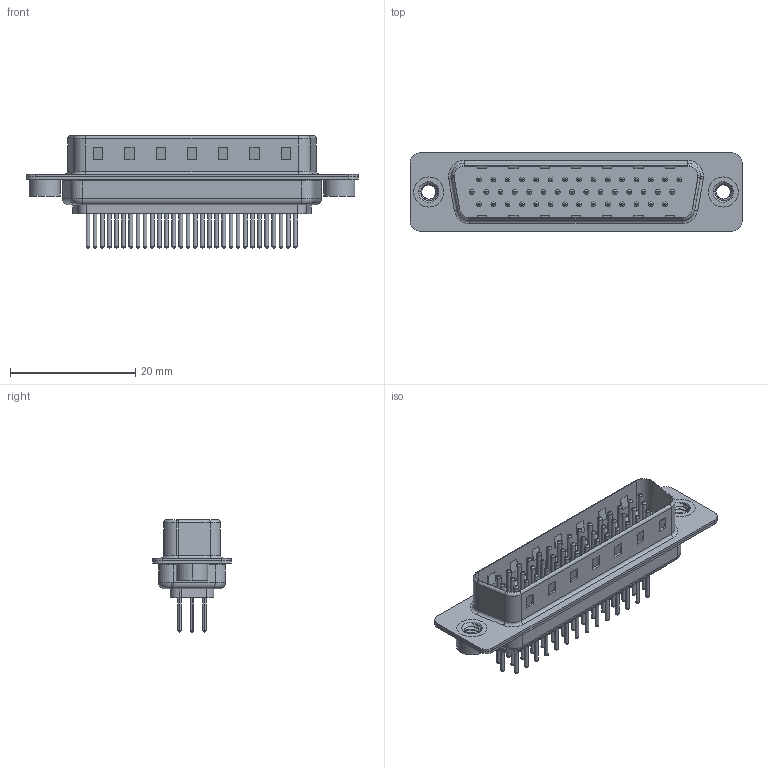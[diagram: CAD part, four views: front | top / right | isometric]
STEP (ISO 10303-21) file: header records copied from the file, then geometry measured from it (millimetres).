
FILE_DESCRIPTION (( 'STEP AP203' ), '1' );
FILE_NAME ('637-M44-630-BT2.STEP', '2018-11-20T01:35:49', ( '' ), ( '' ), 'SwSTEP 2.0', 'SolidWorks 2016', '' );
FILE_SCHEMA (( 'CONFIG_CONTROL_DESIGN' ));
Length unit declared in the file: millimetre
Products named in the file (8): 637M 4-40 Threaded Rivet; 637-M44-630-BT2; 637M Housing_44 Contacts; 637M Shell Front_44 Contacts; 637M Shell Rear_44 Contacts; 637M Contact Row 1_30; 637M Contact Row 2_30; 637M Contact Row 3_30
Assembly tree (49 placements, depth 2):
  637-M44-630-BT2
    637M Housing_44 Contacts
    637M Shell Front_44 Contacts
    637M Shell Rear_44 Contacts
    637M Contact Row 1_30  x15
    637M Contact Row 2_30  x15
    637M Contact Row 3_30  x14
    637M 4-40 Threaded Rivet  x2
Bounding box: 53.05 x 12.5 x 17.9 mm (x, y, z)
Volume: 2828.2 mm3; surface area: 8466.8 mm2
Topology: 49 solids, 49 shells, 2004 faces, 4213 edges, 2538 vertices
Faces by surface type: torus 754, cylinder 753, plane 479, cone 12, bspline 6
Entity records: 26524 total; most frequent: CARTESIAN_POINT 5379, DIRECTION 4412, ORIENTED_EDGE 3672, EDGE_CURVE 1836, AXIS2_PLACEMENT_3D 1792, VERTEX_POINT 1174, EDGE_LOOP 1018, CIRCLE 961
